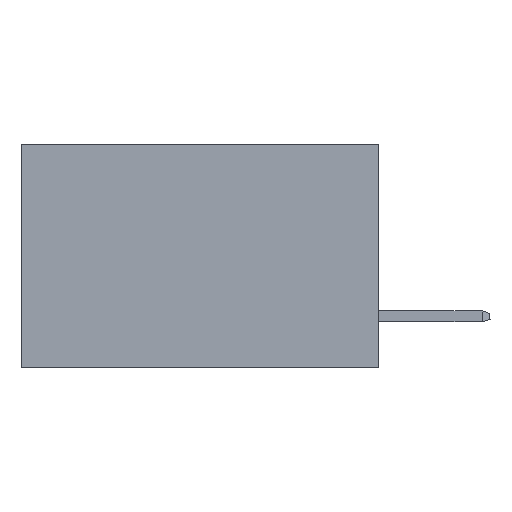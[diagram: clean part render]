
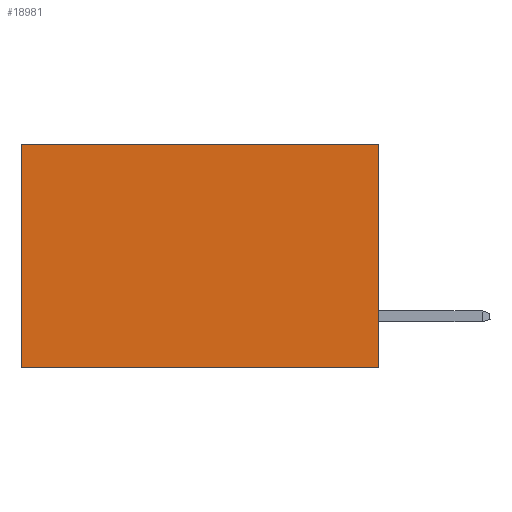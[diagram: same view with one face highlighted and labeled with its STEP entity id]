
A CAD part, left-side view. The second image highlights one B-rep face of the part: STEP entity #18981.
In plain terms, the highlighted planar face has unit normal (-1, 0, 0).
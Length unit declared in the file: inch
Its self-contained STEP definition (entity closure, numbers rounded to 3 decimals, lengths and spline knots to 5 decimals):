
#43 = CARTESIAN_POINT ( 'NONE',  ( 0.277, 0., -0.37 ) ) ;
#304 = ORIENTED_EDGE ( 'NONE', *, *, #15110, .T. ) ;
#326 = EDGE_CURVE ( 'NONE', #22142, #2483, #23474, .T. ) ;
#998 = FACE_OUTER_BOUND ( 'NONE', #5183, .T. ) ;
#2092 = DIRECTION ( 'NONE',  ( 1., 0., 0. ) ) ;
#2355 = LINE ( 'NONE', #11277, #23375 ) ;
#2483 = VERTEX_POINT ( 'NONE', #17570 ) ;
#4064 = AXIS2_PLACEMENT_3D ( 'NONE', #43, #2092, #16458 ) ;
#4513 = VECTOR ( 'NONE', #10725, 39.37008 ) ;
#5183 = EDGE_LOOP ( 'NONE', ( #18384, #24430, #5439, #304 ) ) ;
#5439 = ORIENTED_EDGE ( 'NONE', *, *, #25761, .F. ) ;
#6745 = EDGE_CURVE ( 'NONE', #19986, #2483, #2355, .T. ) ;
#7311 = VECTOR ( 'NONE', #14551, 39.37008 ) ;
#8925 = DIRECTION ( 'NONE',  ( 0., 0., -1. ) ) ;
#9508 = CARTESIAN_POINT ( 'NONE',  ( 0.277, 0., -0.37 ) ) ;
#9609 = CARTESIAN_POINT ( 'NONE',  ( 0.277, 0., -0.37 ) ) ;
#10710 = VECTOR ( 'NONE', #8925, 39.37008 ) ;
#10725 = DIRECTION ( 'NONE',  ( 0., 1., 0. ) ) ;
#10821 = DIRECTION ( 'NONE',  ( 0., 0., -1. ) ) ;
#11277 = CARTESIAN_POINT ( 'NONE',  ( 0.277, 0.59, -0.37 ) ) ;
#12393 = PLANE ( 'NONE',  #4064 ) ;
#14551 = DIRECTION ( 'NONE',  ( 0., 1., 0. ) ) ;
#15110 = EDGE_CURVE ( 'NONE', #21384, #19986, #25472, .T. ) ;
#15888 = CARTESIAN_POINT ( 'NONE',  ( 0.277, 0.59, 0. ) ) ;
#16458 = DIRECTION ( 'NONE',  ( 0., 0., -1. ) ) ;
#16750 = LINE ( 'NONE', #25100, #10710 ) ;
#17570 = CARTESIAN_POINT ( 'NONE',  ( 0.277, 0.59, -0.37 ) ) ;
#18035 = CARTESIAN_POINT ( 'NONE',  ( 0.277, 0., 0. ) ) ;
#18384 = ORIENTED_EDGE ( 'NONE', *, *, #6745, .T. ) ;
#18981 = ADVANCED_FACE ( 'NONE', ( #998 ), #12393, .F. ) ;
#19986 = VERTEX_POINT ( 'NONE', #15888 ) ;
#21384 = VERTEX_POINT ( 'NONE', #18035 ) ;
#22142 = VERTEX_POINT ( 'NONE', #9508 ) ;
#23375 = VECTOR ( 'NONE', #10821, 39.37008 ) ;
#23474 = LINE ( 'NONE', #9609, #7311 ) ;
#24430 = ORIENTED_EDGE ( 'NONE', *, *, #326, .F. ) ;
#24847 = CARTESIAN_POINT ( 'NONE',  ( 0.277, 0., 0. ) ) ;
#25100 = CARTESIAN_POINT ( 'NONE',  ( 0.277, 0., -0.37 ) ) ;
#25472 = LINE ( 'NONE', #24847, #4513 ) ;
#25761 = EDGE_CURVE ( 'NONE', #21384, #22142, #16750, .T. ) ;
